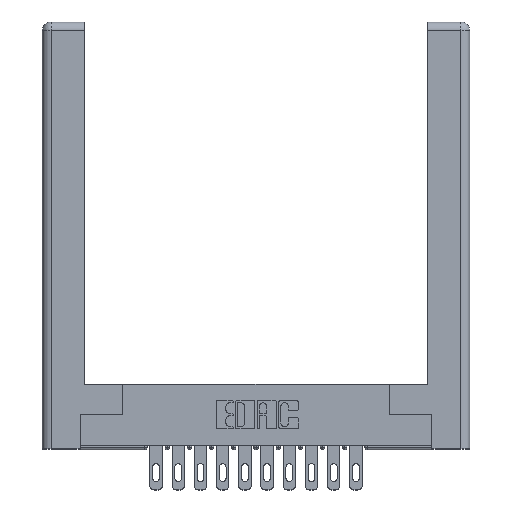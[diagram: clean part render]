
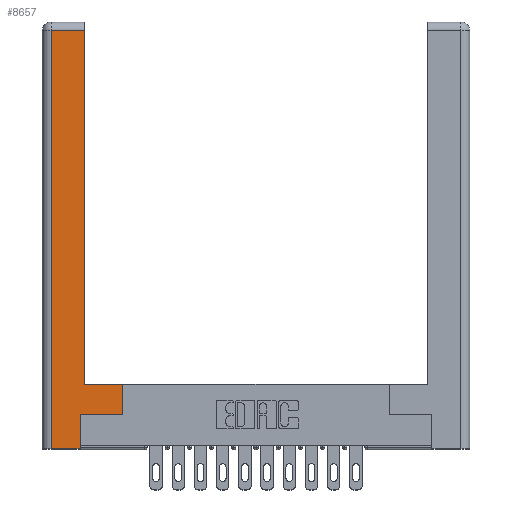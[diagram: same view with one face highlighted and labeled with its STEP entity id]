
A CAD part, top view. The second image highlights one B-rep face of the part: STEP entity #8657.
In plain terms, the highlighted planar face has unit normal (0, 0, 1).
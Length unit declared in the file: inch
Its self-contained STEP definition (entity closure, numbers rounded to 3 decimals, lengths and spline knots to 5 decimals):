
#64 = CARTESIAN_POINT ( 'NONE',  ( 0.0615, 0., 0. ) ) ;
#86 = ORIENTED_EDGE ( 'NONE', *, *, #292, .T. ) ;
#292 = EDGE_CURVE ( 'NONE', #2834, #2684, #7471, .T. ) ;
#631 = CARTESIAN_POINT ( 'NONE',  ( 0.295, 0.45, 0. ) ) ;
#1032 = CARTESIAN_POINT ( 'NONE',  ( 0.565, 0.45, 0. ) ) ;
#1074 = ORIENTED_EDGE ( 'NONE', *, *, #10582, .T. ) ;
#1168 = CARTESIAN_POINT ( 'NONE',  ( 0.565, 0.245, 0. ) ) ;
#1223 = CARTESIAN_POINT ( 'NONE',  ( 0.265, 0.245, 0. ) ) ;
#1769 = EDGE_CURVE ( 'NONE', #2564, #5147, #13452, .T. ) ;
#1823 = CARTESIAN_POINT ( 'NONE',  ( 0.565, 0.245, 0. ) ) ;
#1831 = EDGE_CURVE ( 'NONE', #5587, #2834, #2660, .T. ) ;
#2006 = LINE ( 'NONE', #7705, #4355 ) ;
#2171 = CARTESIAN_POINT ( 'NONE',  ( 0.295, 2.94, 0. ) ) ;
#2257 = DIRECTION ( 'NONE',  ( 1., 0., 0. ) ) ;
#2358 = CARTESIAN_POINT ( 'NONE',  ( 0.0615, 0., 0. ) ) ;
#2564 = VERTEX_POINT ( 'NONE', #1823 ) ;
#2584 = CARTESIAN_POINT ( 'NONE',  ( 0.0615, 2.94, 0. ) ) ;
#2660 = LINE ( 'NONE', #16212, #13861 ) ;
#2684 = VERTEX_POINT ( 'NONE', #2584 ) ;
#2710 = VERTEX_POINT ( 'NONE', #1223 ) ;
#2834 = VERTEX_POINT ( 'NONE', #2171 ) ;
#3108 = ORIENTED_EDGE ( 'NONE', *, *, #4587, .T. ) ;
#3339 = ORIENTED_EDGE ( 'NONE', *, *, #13834, .T. ) ;
#3533 = ORIENTED_EDGE ( 'NONE', *, *, #4395, .T. ) ;
#3581 = ORIENTED_EDGE ( 'NONE', *, *, #1831, .T. ) ;
#3789 = DIRECTION ( 'NONE',  ( 0., 1., 0. ) ) ;
#4355 = VECTOR ( 'NONE', #5290, 39.37008 ) ;
#4395 = EDGE_CURVE ( 'NONE', #5147, #5587, #2006, .T. ) ;
#4535 = LINE ( 'NONE', #4646, #5744 ) ;
#4587 = EDGE_CURVE ( 'NONE', #2710, #2564, #8887, .T. ) ;
#4646 = CARTESIAN_POINT ( 'NONE',  ( 0.265, 0.245, 0. ) ) ;
#4755 = VECTOR ( 'NONE', #2257, 39.37008 ) ;
#4810 = CARTESIAN_POINT ( 'NONE',  ( 0., 0., 0. ) ) ;
#4898 = LINE ( 'NONE', #6557, #12921 ) ;
#5147 = VERTEX_POINT ( 'NONE', #1032 ) ;
#5290 = DIRECTION ( 'NONE',  ( -1., 0., 0. ) ) ;
#5509 = ORIENTED_EDGE ( 'NONE', *, *, #12086, .T. ) ;
#5587 = VERTEX_POINT ( 'NONE', #631 ) ;
#5744 = VECTOR ( 'NONE', #14783, 39.37008 ) ;
#6076 = CARTESIAN_POINT ( 'NONE',  ( 0.565, 0.45, 0. ) ) ;
#6261 = PLANE ( 'NONE',  #13032 ) ;
#6340 = ORIENTED_EDGE ( 'NONE', *, *, #1769, .T. ) ;
#6557 = CARTESIAN_POINT ( 'NONE',  ( 0.265, 0., 0. ) ) ;
#7471 = LINE ( 'NONE', #12069, #12943 ) ;
#7705 = CARTESIAN_POINT ( 'NONE',  ( 0.295, 0.45, 0. ) ) ;
#8420 = LINE ( 'NONE', #64, #15880 ) ;
#8657 = ADVANCED_FACE ( 'NONE', ( #9517 ), #6261, .F. ) ;
#8887 = LINE ( 'NONE', #1168, #4755 ) ;
#9517 = FACE_OUTER_BOUND ( 'NONE', #10888, .T. ) ;
#10582 = EDGE_CURVE ( 'NONE', #11412, #2710, #4535, .T. ) ;
#10888 = EDGE_LOOP ( 'NONE', ( #3581, #86, #3339, #5509, #1074, #3108, #6340, #3533 ) ) ;
#11412 = VERTEX_POINT ( 'NONE', #15037 ) ;
#11896 = DIRECTION ( 'NONE',  ( 1., 0., 0. ) ) ;
#12069 = CARTESIAN_POINT ( 'NONE',  ( 0.0615, 2.94, 0. ) ) ;
#12086 = EDGE_CURVE ( 'NONE', #16289, #11412, #4898, .T. ) ;
#12670 = VECTOR ( 'NONE', #3789, 39.37008 ) ;
#12921 = VECTOR ( 'NONE', #11896, 39.37008 ) ;
#12943 = VECTOR ( 'NONE', #14781, 39.37008 ) ;
#13032 = AXIS2_PLACEMENT_3D ( 'NONE', #4810, #13640, #13754 ) ;
#13452 = LINE ( 'NONE', #6076, #12670 ) ;
#13640 = DIRECTION ( 'NONE',  ( 0., 0., -1. ) ) ;
#13754 = DIRECTION ( 'NONE',  ( -1., 0., 0. ) ) ;
#13834 = EDGE_CURVE ( 'NONE', #2684, #16289, #8420, .T. ) ;
#13861 = VECTOR ( 'NONE', #15305, 39.37008 ) ;
#14781 = DIRECTION ( 'NONE',  ( -1., 0., 0. ) ) ;
#14783 = DIRECTION ( 'NONE',  ( 0., 1., 0. ) ) ;
#15037 = CARTESIAN_POINT ( 'NONE',  ( 0.265, 0., 0. ) ) ;
#15305 = DIRECTION ( 'NONE',  ( 0., 1., 0. ) ) ;
#15880 = VECTOR ( 'NONE', #16271, 39.37008 ) ;
#16212 = CARTESIAN_POINT ( 'NONE',  ( 0.295, 3., 0. ) ) ;
#16271 = DIRECTION ( 'NONE',  ( 0., -1., 0. ) ) ;
#16289 = VERTEX_POINT ( 'NONE', #2358 ) ;
